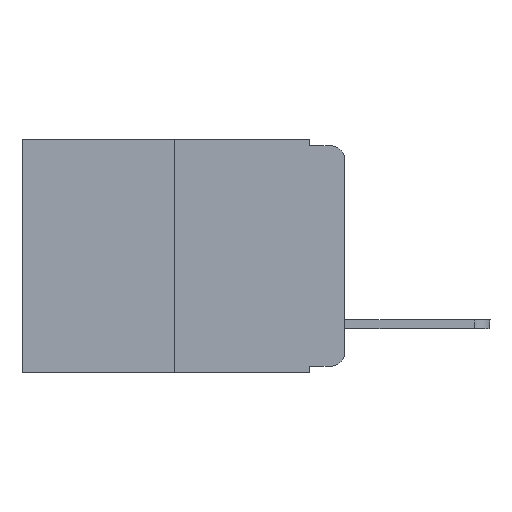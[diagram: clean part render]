
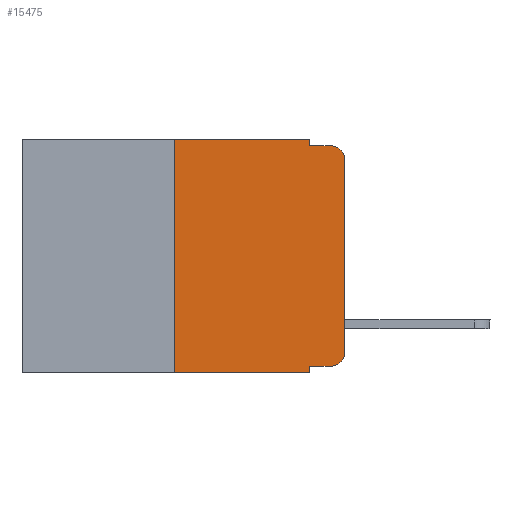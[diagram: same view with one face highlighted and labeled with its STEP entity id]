
A CAD part, left-side view. The second image highlights one B-rep face of the part: STEP entity #15475.
In plain terms, the highlighted planar face has unit normal (-1, 0, 0).
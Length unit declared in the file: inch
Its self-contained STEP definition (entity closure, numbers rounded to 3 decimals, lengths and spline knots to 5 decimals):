
#651 = VERTEX_POINT ( 'NONE', #14644 ) ;
#2181 = CARTESIAN_POINT ( 'NONE',  ( 0., 0., -0.03 ) ) ;
#2614 = CARTESIAN_POINT ( 'NONE',  ( 0., 0.02, -0.03 ) ) ;
#2636 = ORIENTED_EDGE ( 'NONE', *, *, #10959, .F. ) ;
#2858 = LINE ( 'NONE', #7182, #10143 ) ;
#3251 = CARTESIAN_POINT ( 'NONE',  ( 0., 0., -0.313 ) ) ;
#4104 = ORIENTED_EDGE ( 'NONE', *, *, #14832, .T. ) ;
#4329 = ORIENTED_EDGE ( 'NONE', *, *, #12095, .F. ) ;
#4406 = DIRECTION ( 'NONE',  ( 0., 0., -1. ) ) ;
#4549 = DIRECTION ( 'NONE',  ( -1., 0., 0. ) ) ;
#4854 = DIRECTION ( 'NONE',  ( 0., 0., 1. ) ) ;
#4983 = LINE ( 'NONE', #14782, #19489 ) ;
#5336 = DIRECTION ( 'NONE',  ( 0., 0., -1. ) ) ;
#5653 = LINE ( 'NONE', #7831, #19515 ) ;
#5759 = CARTESIAN_POINT ( 'NONE',  ( 0., 0.473, 0. ) ) ;
#5787 = DIRECTION ( 'NONE',  ( 0., 0., -1. ) ) ;
#7030 = CARTESIAN_POINT ( 'NONE',  ( 0., 0.473, -0.343 ) ) ;
#7095 = VERTEX_POINT ( 'NONE', #17217 ) ;
#7182 = CARTESIAN_POINT ( 'NONE',  ( 0., 0.25, 0. ) ) ;
#7263 = LINE ( 'NONE', #11839, #11016 ) ;
#7813 = ORIENTED_EDGE ( 'NONE', *, *, #14554, .F. ) ;
#7831 = CARTESIAN_POINT ( 'NONE',  ( 0., 0.051, 0. ) ) ;
#8240 = CIRCLE ( 'NONE', #10048, 0.02 ) ;
#8634 = VECTOR ( 'NONE', #13746, 39.37008 ) ;
#8822 = DIRECTION ( 'NONE',  ( 0., 0., -1. ) ) ;
#8852 = CARTESIAN_POINT ( 'NONE',  ( 0., 0.051, 0. ) ) ;
#8976 = CIRCLE ( 'NONE', #10132, 0.02 ) ;
#9194 = EDGE_LOOP ( 'NONE', ( #4104, #11973, #4329, #7813, #18796, #18554, #22448, #2636, #13780, #9649 ) ) ;
#9649 = ORIENTED_EDGE ( 'NONE', *, *, #18087, .T. ) ;
#9919 = CARTESIAN_POINT ( 'NONE',  ( 0., 0.25, 0. ) ) ;
#10048 = AXIS2_PLACEMENT_3D ( 'NONE', #17278, #25423, #5336 ) ;
#10132 = AXIS2_PLACEMENT_3D ( 'NONE', #2614, #4549, #8822 ) ;
#10143 = VECTOR ( 'NONE', #11311, 39.37008 ) ;
#10189 = LINE ( 'NONE', #21734, #8634 ) ;
#10257 = CARTESIAN_POINT ( 'NONE',  ( 0., 0.051, 0. ) ) ;
#10566 = CARTESIAN_POINT ( 'NONE',  ( 0., 0.051, -0.343 ) ) ;
#10949 = FACE_OUTER_BOUND ( 'NONE', #9194, .T. ) ;
#10959 = EDGE_CURVE ( 'NONE', #7095, #16619, #18184, .T. ) ;
#11016 = VECTOR ( 'NONE', #13849, 39.37008 ) ;
#11311 = DIRECTION ( 'NONE',  ( 0., 0., 1. ) ) ;
#11839 = CARTESIAN_POINT ( 'NONE',  ( 0., 0.473, 0. ) ) ;
#11973 = ORIENTED_EDGE ( 'NONE', *, *, #21785, .T. ) ;
#12095 = EDGE_CURVE ( 'NONE', #25808, #21698, #10189, .T. ) ;
#12769 = VECTOR ( 'NONE', #13082, 39.37008 ) ;
#13082 = DIRECTION ( 'NONE',  ( 0., -1., 0. ) ) ;
#13145 = EDGE_CURVE ( 'NONE', #651, #22764, #2858, .T. ) ;
#13338 = CARTESIAN_POINT ( 'NONE',  ( 0., 0.051, -0.01 ) ) ;
#13682 = PLANE ( 'NONE',  #19962 ) ;
#13746 = DIRECTION ( 'NONE',  ( 0., -1., 0. ) ) ;
#13780 = ORIENTED_EDGE ( 'NONE', *, *, #23255, .T. ) ;
#13849 = DIRECTION ( 'NONE',  ( 0., -1., 0. ) ) ;
#14130 = VERTEX_POINT ( 'NONE', #3251 ) ;
#14554 = EDGE_CURVE ( 'NONE', #24422, #25808, #5653, .T. ) ;
#14644 = CARTESIAN_POINT ( 'NONE',  ( 0., 0.25, -0.343 ) ) ;
#14782 = CARTESIAN_POINT ( 'NONE',  ( 0., 0., 0. ) ) ;
#14832 = EDGE_CURVE ( 'NONE', #14130, #24916, #4983, .T. ) ;
#15475 = ADVANCED_FACE ( 'NONE', ( #10949 ), #13682, .F. ) ;
#16619 = VERTEX_POINT ( 'NONE', #10566 ) ;
#16961 = CARTESIAN_POINT ( 'NONE',  ( 0., 0.051, -0.333 ) ) ;
#17217 = CARTESIAN_POINT ( 'NONE',  ( 0., 0.051, -0.333 ) ) ;
#17278 = CARTESIAN_POINT ( 'NONE',  ( 0., 0.02, -0.313 ) ) ;
#17518 = CARTESIAN_POINT ( 'NONE',  ( 0., 0.02, -0.333 ) ) ;
#17965 = DIRECTION ( 'NONE',  ( 1., 0., 0. ) ) ;
#18087 = EDGE_CURVE ( 'NONE', #21397, #14130, #8240, .T. ) ;
#18184 = LINE ( 'NONE', #10257, #19454 ) ;
#18358 = EDGE_CURVE ( 'NONE', #22764, #24422, #7263, .T. ) ;
#18554 = ORIENTED_EDGE ( 'NONE', *, *, #13145, .F. ) ;
#18796 = ORIENTED_EDGE ( 'NONE', *, *, #18358, .F. ) ;
#19454 = VECTOR ( 'NONE', #4406, 39.37008 ) ;
#19489 = VECTOR ( 'NONE', #4854, 39.37008 ) ;
#19515 = VECTOR ( 'NONE', #5787, 39.37008 ) ;
#19962 = AXIS2_PLACEMENT_3D ( 'NONE', #5759, #17965, #21842 ) ;
#20404 = CARTESIAN_POINT ( 'NONE',  ( 0., 0.02, -0.01 ) ) ;
#20834 = EDGE_CURVE ( 'NONE', #651, #16619, #22515, .T. ) ;
#21115 = DIRECTION ( 'NONE',  ( 0., -1., 0. ) ) ;
#21397 = VERTEX_POINT ( 'NONE', #17518 ) ;
#21698 = VERTEX_POINT ( 'NONE', #20404 ) ;
#21734 = CARTESIAN_POINT ( 'NONE',  ( 0., 0.051, -0.01 ) ) ;
#21785 = EDGE_CURVE ( 'NONE', #24916, #21698, #8976, .T. ) ;
#21842 = DIRECTION ( 'NONE',  ( 0., 0., -1. ) ) ;
#22448 = ORIENTED_EDGE ( 'NONE', *, *, #20834, .T. ) ;
#22515 = LINE ( 'NONE', #7030, #12769 ) ;
#22764 = VERTEX_POINT ( 'NONE', #9919 ) ;
#23047 = VECTOR ( 'NONE', #21115, 39.37008 ) ;
#23255 = EDGE_CURVE ( 'NONE', #7095, #21397, #23386, .T. ) ;
#23386 = LINE ( 'NONE', #16961, #23047 ) ;
#24422 = VERTEX_POINT ( 'NONE', #8852 ) ;
#24916 = VERTEX_POINT ( 'NONE', #2181 ) ;
#25423 = DIRECTION ( 'NONE',  ( -1., 0., 0. ) ) ;
#25808 = VERTEX_POINT ( 'NONE', #13338 ) ;
